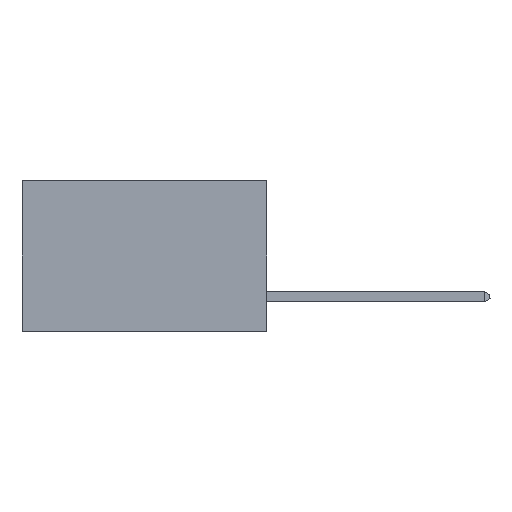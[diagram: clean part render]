
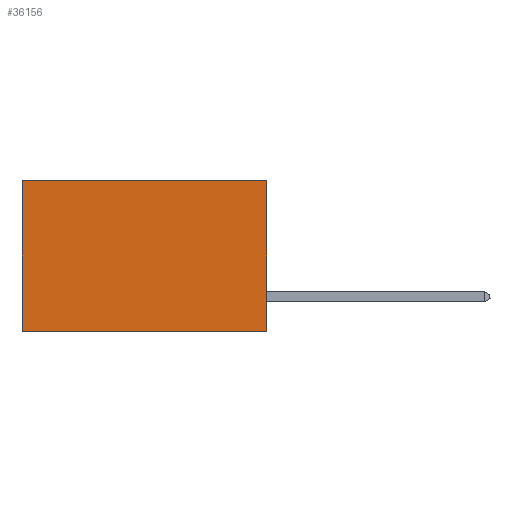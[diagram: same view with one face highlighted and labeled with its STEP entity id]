
A CAD part, left-side view. The second image highlights one B-rep face of the part: STEP entity #36156.
In plain terms, the highlighted planar face has unit normal (-1, 0, 0).
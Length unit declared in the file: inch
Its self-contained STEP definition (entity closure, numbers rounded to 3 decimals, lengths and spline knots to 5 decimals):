
#360 = VERTEX_POINT ( 'NONE', #3481 ) ;
#2967 = FACE_OUTER_BOUND ( 'NONE', #5631, .T. ) ;
#3481 = CARTESIAN_POINT ( 'NONE',  ( 0.2875, 0., -0.37 ) ) ;
#4607 = VECTOR ( 'NONE', #27773, 39.37008 ) ;
#5631 = EDGE_LOOP ( 'NONE', ( #26983, #48185, #30695, #15111 ) ) ;
#5751 = LINE ( 'NONE', #48014, #37634 ) ;
#6484 = EDGE_CURVE ( 'NONE', #8649, #44989, #14419, .T. ) ;
#6879 = DIRECTION ( 'NONE',  ( 0., 1., 0. ) ) ;
#7453 = DIRECTION ( 'NONE',  ( 0., 0., -1. ) ) ;
#8649 = VERTEX_POINT ( 'NONE', #44151 ) ;
#13304 = CARTESIAN_POINT ( 'NONE',  ( 0.2875, 0.6, 0. ) ) ;
#13471 = DIRECTION ( 'NONE',  ( 0., 0., -1. ) ) ;
#13698 = CARTESIAN_POINT ( 'NONE',  ( 0.2875, 0., -0.37 ) ) ;
#13950 = CARTESIAN_POINT ( 'NONE',  ( 0.2875, 0., 0. ) ) ;
#14419 = LINE ( 'NONE', #13304, #4607 ) ;
#15111 = ORIENTED_EDGE ( 'NONE', *, *, #31312, .T. ) ;
#15119 = VECTOR ( 'NONE', #39676, 39.37008 ) ;
#16916 = EDGE_CURVE ( 'NONE', #360, #44989, #18000, .T. ) ;
#17495 = PLANE ( 'NONE',  #37427 ) ;
#18000 = LINE ( 'NONE', #13698, #15119 ) ;
#20487 = CARTESIAN_POINT ( 'NONE',  ( 0.2875, 0., 0. ) ) ;
#22172 = EDGE_CURVE ( 'NONE', #28038, #360, #5751, .T. ) ;
#23172 = VECTOR ( 'NONE', #6879, 39.37008 ) ;
#26983 = ORIENTED_EDGE ( 'NONE', *, *, #6484, .T. ) ;
#27773 = DIRECTION ( 'NONE',  ( 0., 0., -1. ) ) ;
#28038 = VERTEX_POINT ( 'NONE', #20487 ) ;
#28962 = LINE ( 'NONE', #39778, #23172 ) ;
#30695 = ORIENTED_EDGE ( 'NONE', *, *, #22172, .F. ) ;
#31312 = EDGE_CURVE ( 'NONE', #28038, #8649, #28962, .T. ) ;
#35860 = DIRECTION ( 'NONE',  ( 1., 0., 0. ) ) ;
#36156 = ADVANCED_FACE ( 'NONE', ( #2967 ), #17495, .F. ) ;
#37427 = AXIS2_PLACEMENT_3D ( 'NONE', #13950, #35860, #13471 ) ;
#37634 = VECTOR ( 'NONE', #7453, 39.37008 ) ;
#39676 = DIRECTION ( 'NONE',  ( 0., 1., 0. ) ) ;
#39778 = CARTESIAN_POINT ( 'NONE',  ( 0.2875, 0., 0. ) ) ;
#42572 = CARTESIAN_POINT ( 'NONE',  ( 0.2875, 0.6, -0.37 ) ) ;
#44151 = CARTESIAN_POINT ( 'NONE',  ( 0.2875, 0.6, 0. ) ) ;
#44989 = VERTEX_POINT ( 'NONE', #42572 ) ;
#48014 = CARTESIAN_POINT ( 'NONE',  ( 0.2875, 0., 0. ) ) ;
#48185 = ORIENTED_EDGE ( 'NONE', *, *, #16916, .F. ) ;
